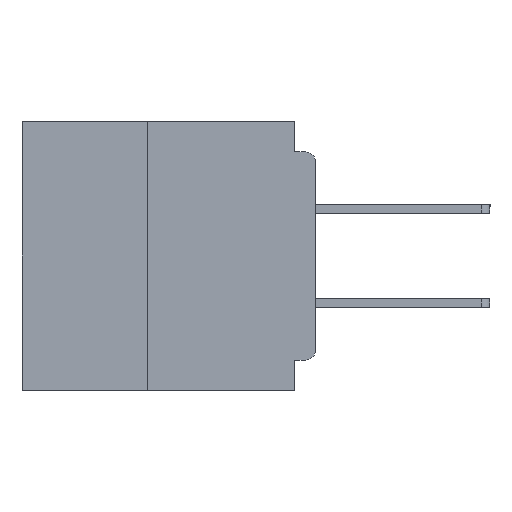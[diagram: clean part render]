
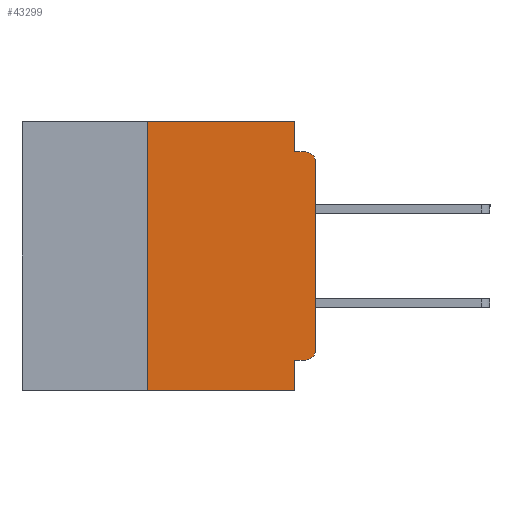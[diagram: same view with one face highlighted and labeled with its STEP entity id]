
A CAD part, left-side view. The second image highlights one B-rep face of the part: STEP entity #43299.
In plain terms, the highlighted planar face has unit normal (-1, 0, 0).
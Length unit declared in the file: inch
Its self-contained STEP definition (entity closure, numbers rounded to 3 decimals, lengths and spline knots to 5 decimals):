
#256 = LINE ( 'NONE', #50276, #44300 ) ;
#1161 = CARTESIAN_POINT ( 'NONE',  ( 0., 0., -0.355 ) ) ;
#2251 = DIRECTION ( 'NONE',  ( 0., 0., -1. ) ) ;
#2588 = VECTOR ( 'NONE', #10954, 39.37008 ) ;
#2777 = CARTESIAN_POINT ( 'NONE',  ( 0., 0.25, -0.4 ) ) ;
#3237 = CARTESIAN_POINT ( 'NONE',  ( 0., 0.015, -0.355 ) ) ;
#3406 = ORIENTED_EDGE ( 'NONE', *, *, #49372, .T. ) ;
#3413 = AXIS2_PLACEMENT_3D ( 'NONE', #7304, #37134, #11608 ) ;
#4363 = VECTOR ( 'NONE', #44716, 39.37008 ) ;
#5046 = EDGE_CURVE ( 'NONE', #19038, #54239, #32544, .T. ) ;
#5683 = LINE ( 'NONE', #14920, #4363 ) ;
#5819 = VERTEX_POINT ( 'NONE', #28573 ) ;
#7304 = CARTESIAN_POINT ( 'NONE',  ( 0., 0.015, -0.06 ) ) ;
#8237 = DIRECTION ( 'NONE',  ( 0., -1., 0. ) ) ;
#8290 = CARTESIAN_POINT ( 'NONE',  ( 0., 0., -0.34 ) ) ;
#8351 = VERTEX_POINT ( 'NONE', #2777 ) ;
#8497 = LINE ( 'NONE', #20944, #27834 ) ;
#9057 = ORIENTED_EDGE ( 'NONE', *, *, #5046, .T. ) ;
#9557 = VERTEX_POINT ( 'NONE', #37026 ) ;
#9825 = VECTOR ( 'NONE', #45412, 39.37008 ) ;
#10056 = EDGE_LOOP ( 'NONE', ( #3406, #30702, #26536, #22587, #26365, #27456, #27690, #47224, #31115, #9057 ) ) ;
#10235 = LINE ( 'NONE', #17960, #42899 ) ;
#10952 = VERTEX_POINT ( 'NONE', #20846 ) ;
#10954 = DIRECTION ( 'NONE',  ( 0., 0., 1. ) ) ;
#11076 = CARTESIAN_POINT ( 'NONE',  ( 0., 0.031, -0.4 ) ) ;
#11217 = LINE ( 'NONE', #1161, #21242 ) ;
#11431 = PLANE ( 'NONE',  #24399 ) ;
#11608 = DIRECTION ( 'NONE',  ( 0., 0., -1. ) ) ;
#12830 = CARTESIAN_POINT ( 'NONE',  ( 0., 0.031, 0. ) ) ;
#13452 = FACE_OUTER_BOUND ( 'NONE', #10056, .T. ) ;
#13978 = LINE ( 'NONE', #32202, #2588 ) ;
#14920 = CARTESIAN_POINT ( 'NONE',  ( 0., 0.031, -0.4 ) ) ;
#15703 = DIRECTION ( 'NONE',  ( 1., 0., 0. ) ) ;
#17960 = CARTESIAN_POINT ( 'NONE',  ( 0., 0., -0.045 ) ) ;
#19038 = VERTEX_POINT ( 'NONE', #3237 ) ;
#20537 = DIRECTION ( 'NONE',  ( 0., 0., -1. ) ) ;
#20846 = CARTESIAN_POINT ( 'NONE',  ( 0., 0.015, -0.045 ) ) ;
#20944 = CARTESIAN_POINT ( 'NONE',  ( 0., 0.437, -0.4 ) ) ;
#21242 = VECTOR ( 'NONE', #31043, 39.37008 ) ;
#22392 = EDGE_CURVE ( 'NONE', #36787, #23689, #5683, .T. ) ;
#22587 = ORIENTED_EDGE ( 'NONE', *, *, #50918, .F. ) ;
#23689 = VERTEX_POINT ( 'NONE', #11076 ) ;
#23800 = VERTEX_POINT ( 'NONE', #49757 ) ;
#24399 = AXIS2_PLACEMENT_3D ( 'NONE', #41242, #15703, #45464 ) ;
#26365 = ORIENTED_EDGE ( 'NONE', *, *, #34381, .F. ) ;
#26536 = ORIENTED_EDGE ( 'NONE', *, *, #37259, .F. ) ;
#26908 = EDGE_CURVE ( 'NONE', #19038, #36787, #11217, .T. ) ;
#27456 = ORIENTED_EDGE ( 'NONE', *, *, #48052, .F. ) ;
#27690 = ORIENTED_EDGE ( 'NONE', *, *, #28151, .T. ) ;
#27834 = VECTOR ( 'NONE', #8237, 39.37008 ) ;
#27910 = DIRECTION ( 'NONE',  ( -1., 0., 0. ) ) ;
#27998 = EDGE_CURVE ( 'NONE', #5819, #10952, #46458, .T. ) ;
#28151 = EDGE_CURVE ( 'NONE', #8351, #23689, #8497, .T. ) ;
#28573 = CARTESIAN_POINT ( 'NONE',  ( 0., 0., -0.06 ) ) ;
#30702 = ORIENTED_EDGE ( 'NONE', *, *, #27998, .T. ) ;
#31043 = DIRECTION ( 'NONE',  ( 0., 1., 0. ) ) ;
#31115 = ORIENTED_EDGE ( 'NONE', *, *, #26908, .F. ) ;
#31827 = LINE ( 'NONE', #46500, #53074 ) ;
#32000 = CARTESIAN_POINT ( 'NONE',  ( 0., 0.031, -0.355 ) ) ;
#32202 = CARTESIAN_POINT ( 'NONE',  ( 0., 0.25, -0.4 ) ) ;
#32544 = CIRCLE ( 'NONE', #37632, 0.015 ) ;
#33873 = LINE ( 'NONE', #41186, #9825 ) ;
#34381 = EDGE_CURVE ( 'NONE', #23800, #53626, #31827, .T. ) ;
#34926 = DIRECTION ( 'NONE',  ( 0., -1., 0. ) ) ;
#36787 = VERTEX_POINT ( 'NONE', #32000 ) ;
#37026 = CARTESIAN_POINT ( 'NONE',  ( 0., 0.031, -0.045 ) ) ;
#37134 = DIRECTION ( 'NONE',  ( -1., 0., 0. ) ) ;
#37259 = EDGE_CURVE ( 'NONE', #9557, #10952, #10235, .T. ) ;
#37632 = AXIS2_PLACEMENT_3D ( 'NONE', #53321, #27910, #2251 ) ;
#41186 = CARTESIAN_POINT ( 'NONE',  ( 0., 0., 0. ) ) ;
#41242 = CARTESIAN_POINT ( 'NONE',  ( 0., 0.437, 0. ) ) ;
#42899 = VECTOR ( 'NONE', #34926, 39.37008 ) ;
#43299 = ADVANCED_FACE ( 'NONE', ( #13452 ), #11431, .F. ) ;
#44300 = VECTOR ( 'NONE', #20537, 39.37008 ) ;
#44716 = DIRECTION ( 'NONE',  ( 0., 0., -1. ) ) ;
#45412 = DIRECTION ( 'NONE',  ( 0., 0., 1. ) ) ;
#45464 = DIRECTION ( 'NONE',  ( 0., 0., -1. ) ) ;
#46458 = CIRCLE ( 'NONE', #3413, 0.015 ) ;
#46500 = CARTESIAN_POINT ( 'NONE',  ( 0., 0.437, 0. ) ) ;
#47224 = ORIENTED_EDGE ( 'NONE', *, *, #22392, .F. ) ;
#48052 = EDGE_CURVE ( 'NONE', #8351, #23800, #13978, .T. ) ;
#49372 = EDGE_CURVE ( 'NONE', #54239, #5819, #33873, .T. ) ;
#49757 = CARTESIAN_POINT ( 'NONE',  ( 0., 0.25, 0. ) ) ;
#50276 = CARTESIAN_POINT ( 'NONE',  ( 0., 0.031, 0. ) ) ;
#50784 = DIRECTION ( 'NONE',  ( 0., -1., 0. ) ) ;
#50918 = EDGE_CURVE ( 'NONE', #53626, #9557, #256, .T. ) ;
#53074 = VECTOR ( 'NONE', #50784, 39.37008 ) ;
#53321 = CARTESIAN_POINT ( 'NONE',  ( 0., 0.015, -0.34 ) ) ;
#53626 = VERTEX_POINT ( 'NONE', #12830 ) ;
#54239 = VERTEX_POINT ( 'NONE', #8290 ) ;
